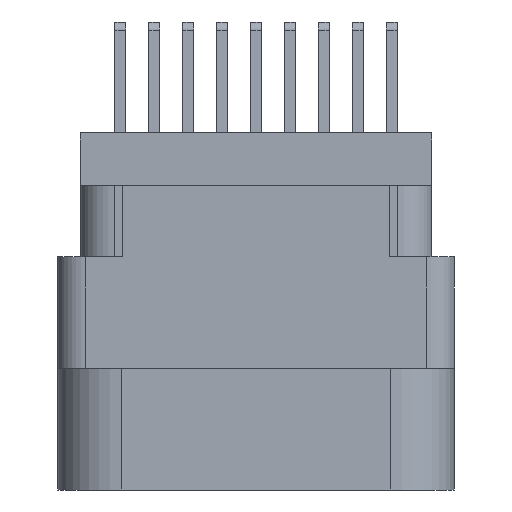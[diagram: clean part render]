
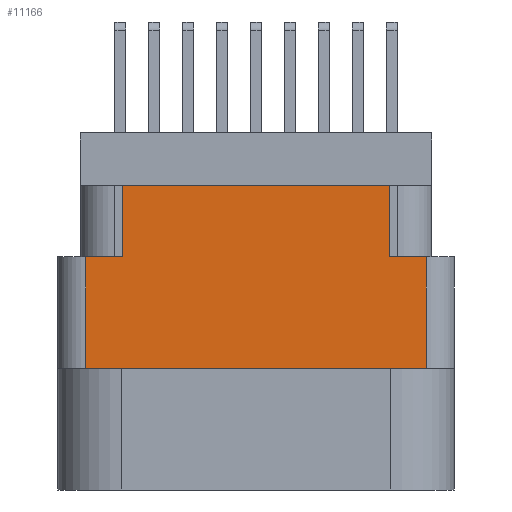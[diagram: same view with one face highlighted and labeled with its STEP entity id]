
A CAD part, left-side view. The second image highlights one B-rep face of the part: STEP entity #11166.
In plain terms, the highlighted planar face has unit normal (-1, 0, 0).
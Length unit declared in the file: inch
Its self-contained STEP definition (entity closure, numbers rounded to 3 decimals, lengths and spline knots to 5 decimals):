
#366 = VECTOR ( 'NONE', #13065, 39.37008 ) ;
#370 = DIRECTION ( 'NONE',  ( 0., 0., 1. ) ) ;
#1321 = VECTOR ( 'NONE', #20212, 39.37008 ) ;
#2847 = EDGE_CURVE ( 'NONE', #8115, #37420, #44695, .T. ) ;
#3358 = ORIENTED_EDGE ( 'NONE', *, *, #23616, .F. ) ;
#3648 = VECTOR ( 'NONE', #8046, 39.37008 ) ;
#6129 = CARTESIAN_POINT ( 'NONE',  ( -1.2955, -0.376, -0.789 ) ) ;
#7748 = ORIENTED_EDGE ( 'NONE', *, *, #14173, .T. ) ;
#8046 = DIRECTION ( 'NONE',  ( 0., -1., 0. ) ) ;
#8115 = VERTEX_POINT ( 'NONE', #24015 ) ;
#9462 = VECTOR ( 'NONE', #370, 39.37008 ) ;
#9599 = PLANE ( 'NONE',  #22536 ) ;
#9614 = CARTESIAN_POINT ( 'NONE',  ( -1.2955, 0.376, -0.789 ) ) ;
#9751 = CARTESIAN_POINT ( 'NONE',  ( -1.2955, -0.438, -0.789 ) ) ;
#10823 = CARTESIAN_POINT ( 'NONE',  ( -1.2955, -0.376, -0.274 ) ) ;
#10997 = CARTESIAN_POINT ( 'NONE',  ( -1.2955, -0.296, -0.274 ) ) ;
#11166 = ADVANCED_FACE ( 'NONE', ( #34626 ), #9599, .T. ) ;
#12851 = VERTEX_POINT ( 'NONE', #13332 ) ;
#13065 = DIRECTION ( 'NONE',  ( 0., -1., 0. ) ) ;
#13103 = EDGE_CURVE ( 'NONE', #18729, #12851, #37175, .T. ) ;
#13148 = CARTESIAN_POINT ( 'NONE',  ( -1.2955, -0.376, -0.52 ) ) ;
#13320 = EDGE_CURVE ( 'NONE', #25674, #25960, #42728, .T. ) ;
#13332 = CARTESIAN_POINT ( 'NONE',  ( -1.2955, 0.296, -0.274 ) ) ;
#14173 = EDGE_CURVE ( 'NONE', #18729, #23278, #45355, .T. ) ;
#14498 = EDGE_CURVE ( 'NONE', #42238, #23278, #42007, .T. ) ;
#17813 = VECTOR ( 'NONE', #39556, 39.37008 ) ;
#18373 = ORIENTED_EDGE ( 'NONE', *, *, #14498, .F. ) ;
#18729 = VERTEX_POINT ( 'NONE', #33894 ) ;
#20212 = DIRECTION ( 'NONE',  ( 0., 0., -1. ) ) ;
#20367 = ORIENTED_EDGE ( 'NONE', *, *, #13320, .F. ) ;
#22536 = AXIS2_PLACEMENT_3D ( 'NONE', #9751, #44676, #44985 ) ;
#23278 = VERTEX_POINT ( 'NONE', #25534 ) ;
#23616 = EDGE_CURVE ( 'NONE', #12851, #25674, #25376, .T. ) ;
#23894 = DIRECTION ( 'NONE',  ( 0., 0., 1. ) ) ;
#24015 = CARTESIAN_POINT ( 'NONE',  ( -1.2955, -0.296, -0.274 ) ) ;
#25319 = LINE ( 'NONE', #6129, #32474 ) ;
#25376 = LINE ( 'NONE', #44921, #29258 ) ;
#25534 = CARTESIAN_POINT ( 'NONE',  ( -1.2955, 0.376, -0.52 ) ) ;
#25546 = CARTESIAN_POINT ( 'NONE',  ( -1.2955, 0., -0.52 ) ) ;
#25647 = ORIENTED_EDGE ( 'NONE', *, *, #43909, .T. ) ;
#25674 = VERTEX_POINT ( 'NONE', #32305 ) ;
#25960 = VERTEX_POINT ( 'NONE', #31960 ) ;
#27043 = CARTESIAN_POINT ( 'NONE',  ( -1.2955, 0., -0.274 ) ) ;
#27336 = CARTESIAN_POINT ( 'NONE',  ( -1.2955, 0., -0.274 ) ) ;
#28128 = EDGE_CURVE ( 'NONE', #8115, #25960, #39139, .T. ) ;
#28328 = DIRECTION ( 'NONE',  ( 0., 0., 1. ) ) ;
#29258 = VECTOR ( 'NONE', #28328, 39.37008 ) ;
#30351 = ORIENTED_EDGE ( 'NONE', *, *, #13103, .F. ) ;
#31960 = CARTESIAN_POINT ( 'NONE',  ( -1.2955, -0.296, -0.117 ) ) ;
#32305 = CARTESIAN_POINT ( 'NONE',  ( -1.2955, 0.296, -0.117 ) ) ;
#32474 = VECTOR ( 'NONE', #23894, 39.37008 ) ;
#33506 = EDGE_LOOP ( 'NONE', ( #30351, #7748, #18373, #25647, #33876, #37627, #20367, #3358 ) ) ;
#33876 = ORIENTED_EDGE ( 'NONE', *, *, #2847, .F. ) ;
#33894 = CARTESIAN_POINT ( 'NONE',  ( -1.2955, 0.376, -0.274 ) ) ;
#34626 = FACE_OUTER_BOUND ( 'NONE', #33506, .T. ) ;
#35316 = VECTOR ( 'NONE', #44424, 39.37008 ) ;
#35870 = CARTESIAN_POINT ( 'NONE',  ( -1.2955, 0.438, -0.117 ) ) ;
#37175 = LINE ( 'NONE', #27043, #366 ) ;
#37420 = VERTEX_POINT ( 'NONE', #10823 ) ;
#37627 = ORIENTED_EDGE ( 'NONE', *, *, #28128, .T. ) ;
#39139 = LINE ( 'NONE', #10997, #9462 ) ;
#39556 = DIRECTION ( 'NONE',  ( 0., 1., 0. ) ) ;
#42007 = LINE ( 'NONE', #25546, #17813 ) ;
#42238 = VERTEX_POINT ( 'NONE', #13148 ) ;
#42728 = LINE ( 'NONE', #35870, #3648 ) ;
#43909 = EDGE_CURVE ( 'NONE', #42238, #37420, #25319, .T. ) ;
#44424 = DIRECTION ( 'NONE',  ( 0., -1., 0. ) ) ;
#44676 = DIRECTION ( 'NONE',  ( -1., 0., 0. ) ) ;
#44695 = LINE ( 'NONE', #27336, #35316 ) ;
#44921 = CARTESIAN_POINT ( 'NONE',  ( -1.2955, 0.296, -0.274 ) ) ;
#44985 = DIRECTION ( 'NONE',  ( 0., 0., 1. ) ) ;
#45355 = LINE ( 'NONE', #9614, #1321 ) ;
